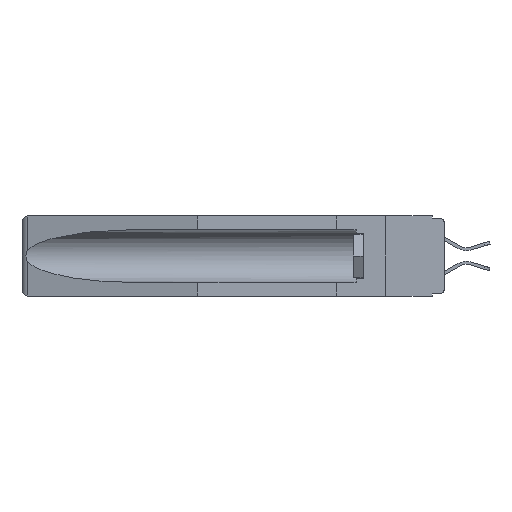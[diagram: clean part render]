
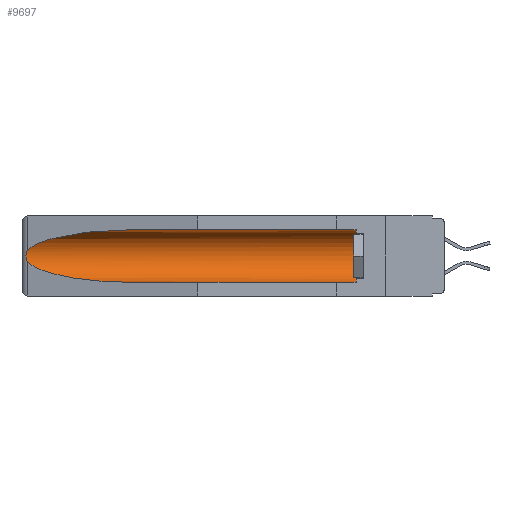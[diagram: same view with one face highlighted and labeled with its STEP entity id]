
A CAD part, left-side view. The second image highlights one B-rep face of the part: STEP entity #9697.
In plain terms, the highlighted cylindrical face has radius 2.857 mm (diameter 5.715 mm), a partial arc.
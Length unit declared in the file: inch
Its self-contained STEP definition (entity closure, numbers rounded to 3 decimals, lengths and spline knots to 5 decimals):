
#249 = AXIS2_PLACEMENT_3D ( 'NONE', #18868, #8576, #3331 ) ;
#391 = CARTESIAN_POINT ( 'NONE',  ( 0.2675, 1.53308, -0.16763 ) ) ;
#599 = EDGE_CURVE ( 'NONE', #22607, #12895, #6991, .T. ) ;
#780 = VECTOR ( 'NONE', #16510, 39.37008 ) ;
#1144 = ORIENTED_EDGE ( 'NONE', *, *, #599, .T. ) ;
#1237 = CARTESIAN_POINT ( 'NONE',  ( 0.25451, 1.48313, -0.09465 ) ) ;
#1466 = CYLINDRICAL_SURFACE ( 'NONE', #249, 0.1125 ) ;
#1828 = EDGE_CURVE ( 'NONE', #19108, #12895, #22935, .T. ) ;
#2384 = CARTESIAN_POINT ( 'NONE',  ( 0.26537, 1.52718, -0.19328 ) ) ;
#3331 = DIRECTION ( 'NONE',  ( 0., 0., 1. ) ) ;
#3620 = DIRECTION ( 'NONE',  ( 0., -1., 0. ) ) ;
#3739 = DIRECTION ( 'NONE',  ( 0., 0., 1. ) ) ;
#4014 = CARTESIAN_POINT ( 'NONE',  ( 0.2675, 1.53308, -0.17534 ) ) ;
#4812 = VERTEX_POINT ( 'NONE', #6148 ) ;
#5083 = FACE_OUTER_BOUND ( 'NONE', #14481, .T. ) ;
#5517 =( BOUNDED_CURVE ( )  B_SPLINE_CURVE ( 3, ( #6709, #18983, #1237, #15461 ),
 .UNSPECIFIED., .F., .F. ) 
 B_SPLINE_CURVE_WITH_KNOTS ( ( 4, 4 ),
 ( 4.71239, 6.08839 ),
 .UNSPECIFIED. ) 
 CURVE ( )  GEOMETRIC_REPRESENTATION_ITEM ( )  RATIONAL_B_SPLINE_CURVE ( ( 1., 0.848, 0.848, 1. ) ) 
 REPRESENTATION_ITEM ( '' )  );
#5644 = CARTESIAN_POINT ( 'NONE',  ( 0.26597, 1.5296, -0.19026 ) ) ;
#6148 = CARTESIAN_POINT ( 'NONE',  ( 0.155, 0.126, -0.059 ) ) ;
#6709 = CARTESIAN_POINT ( 'NONE',  ( 0.155, 1.07973, -0.059 ) ) ;
#6991 =( BOUNDED_CURVE ( )  B_SPLINE_CURVE ( 3, ( #2384, #16609, #9275, #12649 ),
 .UNSPECIFIED., .F., .F. ) 
 B_SPLINE_CURVE_WITH_KNOTS ( ( 4, 4 ),
 ( 0.1948, 1.5708 ),
 .UNSPECIFIED. ) 
 CURVE ( )  GEOMETRIC_REPRESENTATION_ITEM ( )  RATIONAL_B_SPLINE_CURVE ( ( 1., 0.848, 0.848, 1. ) ) 
 REPRESENTATION_ITEM ( '' )  );
#7470 = ORIENTED_EDGE ( 'NONE', *, *, #11180, .T. ) ;
#7733 = CARTESIAN_POINT ( 'NONE',  ( 0.2673, 1.53269, -0.17917 ) ) ;
#8075 = VERTEX_POINT ( 'NONE', #15393 ) ;
#8256 = ORIENTED_EDGE ( 'NONE', *, *, #22812, .T. ) ;
#8555 = CARTESIAN_POINT ( 'NONE',  ( 0.155, 1.07973, -0.284 ) ) ;
#8576 = DIRECTION ( 'NONE',  ( 0., 1., 0. ) ) ;
#9105 = CARTESIAN_POINT ( 'NONE',  ( 0.155, 0.126, -0.1715 ) ) ;
#9275 = CARTESIAN_POINT ( 'NONE',  ( 0.21114, 1.30732, -0.284 ) ) ;
#9697 = ADVANCED_FACE ( 'NONE', ( #5083 ), #1466, .F. ) ;
#10855 = ORIENTED_EDGE ( 'NONE', *, *, #22442, .T. ) ;
#10886 = CARTESIAN_POINT ( 'NONE',  ( 0.26654, 1.53092, -0.15636 ) ) ;
#11180 = EDGE_CURVE ( 'NONE', #18254, #8075, #5517, .T. ) ;
#11240 = CARTESIAN_POINT ( 'NONE',  ( 0.26655, 1.53094, -0.18657 ) ) ;
#11518 = AXIS2_PLACEMENT_3D ( 'NONE', #9105, #3620, #3739 ) ;
#12119 = EDGE_CURVE ( 'NONE', #19108, #4812, #19332, .T. ) ;
#12649 = CARTESIAN_POINT ( 'NONE',  ( 0.155, 1.07973, -0.284 ) ) ;
#12895 = VERTEX_POINT ( 'NONE', #8555 ) ;
#13572 = CARTESIAN_POINT ( 'NONE',  ( 0.26537, 1.52718, -0.19328 ) ) ;
#14481 = EDGE_LOOP ( 'NONE', ( #7470, #8256, #1144, #18138, #15869, #10855 ) ) ;
#15393 = CARTESIAN_POINT ( 'NONE',  ( 0.26537, 1.52718, -0.14972 ) ) ;
#15454 = CARTESIAN_POINT ( 'NONE',  ( 0.155, 0.126, -0.284 ) ) ;
#15461 = CARTESIAN_POINT ( 'NONE',  ( 0.26537, 1.52718, -0.14972 ) ) ;
#15869 = ORIENTED_EDGE ( 'NONE', *, *, #12119, .T. ) ;
#16247 = CARTESIAN_POINT ( 'NONE',  ( 0.2673, 1.5327, -0.16383 ) ) ;
#16397 = LINE ( 'NONE', #20134, #780 ) ;
#16510 = DIRECTION ( 'NONE',  ( 0., 1., 0. ) ) ;
#16609 = CARTESIAN_POINT ( 'NONE',  ( 0.25451, 1.48313, -0.24835 ) ) ;
#17440 = CARTESIAN_POINT ( 'NONE',  ( 0.155, -0.30754, -0.284 ) ) ;
#17480 = B_SPLINE_CURVE_WITH_KNOTS ( 'NONE', 3,
 ( #18256, #19993, #10886, #16247, #391, #4014, #7733, #11240, #5644, #18132 ),
 .UNSPECIFIED., .F., .F.,
 ( 4, 2, 2, 2, 4 ),
 ( 0., 0.00029, 0.00058, 0.00087, 0.00117 ),
 .UNSPECIFIED. ) ;
#17494 = CARTESIAN_POINT ( 'NONE',  ( 0.155, 1.07973, -0.059 ) ) ;
#17786 = DIRECTION ( 'NONE',  ( 0., 1., 0. ) ) ;
#18132 = CARTESIAN_POINT ( 'NONE',  ( 0.26537, 1.52718, -0.19328 ) ) ;
#18138 = ORIENTED_EDGE ( 'NONE', *, *, #1828, .F. ) ;
#18254 = VERTEX_POINT ( 'NONE', #17494 ) ;
#18256 = CARTESIAN_POINT ( 'NONE',  ( 0.26537, 1.52718, -0.14972 ) ) ;
#18868 = CARTESIAN_POINT ( 'NONE',  ( 0.155, -0.30754, -0.1715 ) ) ;
#18983 = CARTESIAN_POINT ( 'NONE',  ( 0.21114, 1.30732, -0.059 ) ) ;
#19108 = VERTEX_POINT ( 'NONE', #15454 ) ;
#19332 = CIRCLE ( 'NONE', #11518, 0.1125 ) ;
#19993 = CARTESIAN_POINT ( 'NONE',  ( 0.26597, 1.52961, -0.15275 ) ) ;
#20134 = CARTESIAN_POINT ( 'NONE',  ( 0.155, -0.30754, -0.059 ) ) ;
#21150 = VECTOR ( 'NONE', #17786, 39.37008 ) ;
#22442 = EDGE_CURVE ( 'NONE', #4812, #18254, #16397, .T. ) ;
#22607 = VERTEX_POINT ( 'NONE', #13572 ) ;
#22812 = EDGE_CURVE ( 'NONE', #8075, #22607, #17480, .T. ) ;
#22935 = LINE ( 'NONE', #17440, #21150 ) ;
